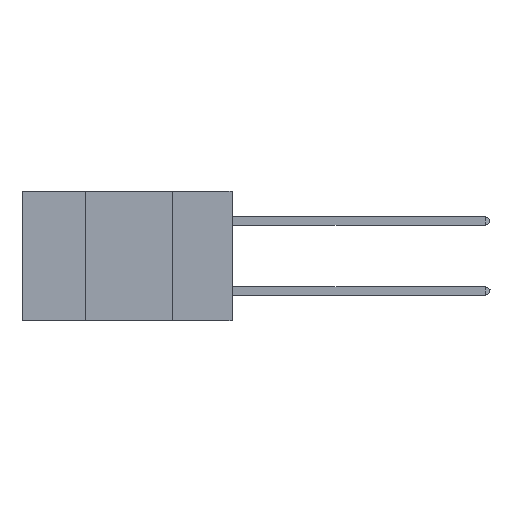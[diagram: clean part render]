
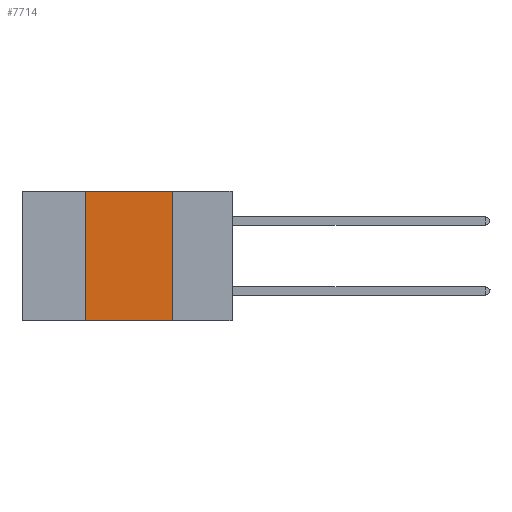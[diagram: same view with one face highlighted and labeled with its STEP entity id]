
A CAD part, left-side view. The second image highlights one B-rep face of the part: STEP entity #7714.
In plain terms, the highlighted planar face has unit normal (-1, 0, 0).
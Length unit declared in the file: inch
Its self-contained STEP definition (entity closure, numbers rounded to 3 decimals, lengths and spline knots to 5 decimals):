
#377 = LINE ( 'NONE', #5049, #10944 ) ;
#1485 = CARTESIAN_POINT ( 'NONE',  ( 0., 0.42, -0.37 ) ) ;
#2401 = DIRECTION ( 'NONE',  ( 1., 0., 0. ) ) ;
#2822 = ORIENTED_EDGE ( 'NONE', *, *, #4447, .F. ) ;
#2924 = DIRECTION ( 'NONE',  ( 0., -1., 0. ) ) ;
#2993 = PLANE ( 'NONE',  #8776 ) ;
#3081 = VERTEX_POINT ( 'NONE', #5438 ) ;
#3968 = LINE ( 'NONE', #6181, #4916 ) ;
#4029 = DIRECTION ( 'NONE',  ( 0., 0., -1. ) ) ;
#4169 = CARTESIAN_POINT ( 'NONE',  ( 0., 0.17, -0.37 ) ) ;
#4447 = EDGE_CURVE ( 'NONE', #6661, #3081, #13291, .T. ) ;
#4916 = VECTOR ( 'NONE', #8356, 39.37008 ) ;
#4982 = DIRECTION ( 'NONE',  ( 0., 0., -1. ) ) ;
#5049 = CARTESIAN_POINT ( 'NONE',  ( 0., 0.17, 0. ) ) ;
#5438 = CARTESIAN_POINT ( 'NONE',  ( 0., 0.42, 0. ) ) ;
#6058 = VERTEX_POINT ( 'NONE', #12855 ) ;
#6181 = CARTESIAN_POINT ( 'NONE',  ( 0., 0.6, -0.37 ) ) ;
#6661 = VERTEX_POINT ( 'NONE', #1485 ) ;
#7267 = CARTESIAN_POINT ( 'NONE',  ( 0., 0.6, 0. ) ) ;
#7714 = ADVANCED_FACE ( 'NONE', ( #11857 ), #2993, .F. ) ;
#8039 = EDGE_CURVE ( 'NONE', #6058, #12081, #377, .T. ) ;
#8093 = CARTESIAN_POINT ( 'NONE',  ( 0., 0.42, 0. ) ) ;
#8302 = ORIENTED_EDGE ( 'NONE', *, *, #12085, .T. ) ;
#8310 = ORIENTED_EDGE ( 'NONE', *, *, #8039, .F. ) ;
#8356 = DIRECTION ( 'NONE',  ( 0., -1., 0. ) ) ;
#8776 = AXIS2_PLACEMENT_3D ( 'NONE', #7267, #2401, #4982 ) ;
#9031 = LINE ( 'NONE', #11146, #9701 ) ;
#9419 = EDGE_LOOP ( 'NONE', ( #8310, #11700, #2822, #8302 ) ) ;
#9701 = VECTOR ( 'NONE', #2924, 39.37008 ) ;
#10342 = DIRECTION ( 'NONE',  ( 0., 0., 1. ) ) ;
#10944 = VECTOR ( 'NONE', #4029, 39.37008 ) ;
#11146 = CARTESIAN_POINT ( 'NONE',  ( 0., 0.6, 0. ) ) ;
#11700 = ORIENTED_EDGE ( 'NONE', *, *, #11764, .F. ) ;
#11764 = EDGE_CURVE ( 'NONE', #3081, #6058, #9031, .T. ) ;
#11857 = FACE_OUTER_BOUND ( 'NONE', #9419, .T. ) ;
#12081 = VERTEX_POINT ( 'NONE', #4169 ) ;
#12085 = EDGE_CURVE ( 'NONE', #6661, #12081, #3968, .T. ) ;
#12645 = VECTOR ( 'NONE', #10342, 39.37008 ) ;
#12855 = CARTESIAN_POINT ( 'NONE',  ( 0., 0.17, 0. ) ) ;
#13291 = LINE ( 'NONE', #8093, #12645 ) ;
